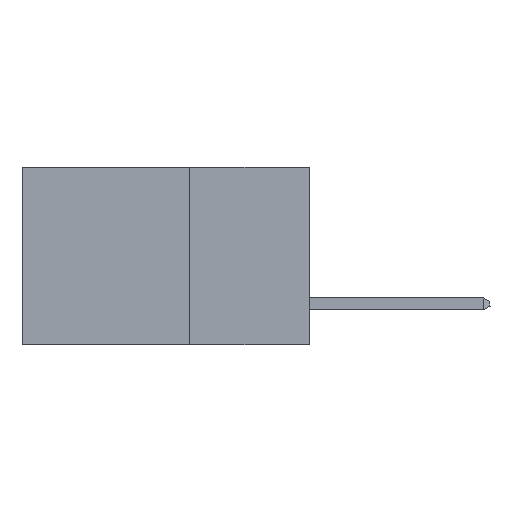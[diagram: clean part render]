
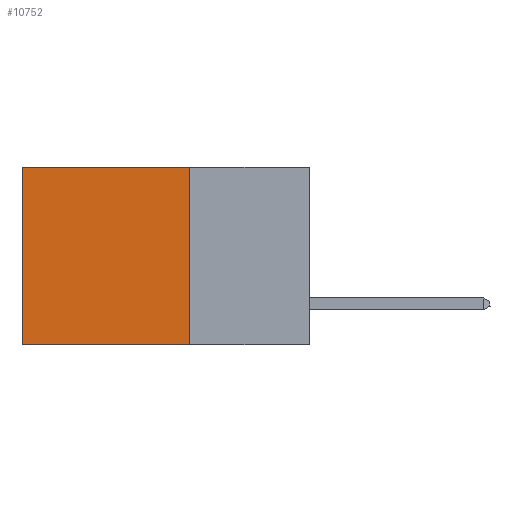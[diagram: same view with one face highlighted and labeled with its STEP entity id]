
A CAD part, left-side view. The second image highlights one B-rep face of the part: STEP entity #10752.
In plain terms, the highlighted planar face has unit normal (-1, 0, 0).
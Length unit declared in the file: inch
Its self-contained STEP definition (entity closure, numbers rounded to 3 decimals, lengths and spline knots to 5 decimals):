
#923 = LINE ( 'NONE', #5842, #4496 ) ;
#1606 = VECTOR ( 'NONE', #9957, 39.37008 ) ;
#1631 = CARTESIAN_POINT ( 'NONE',  ( 0.2875, 0.6, 0. ) ) ;
#1656 = CARTESIAN_POINT ( 'NONE',  ( 0.2875, 0.25, 0. ) ) ;
#2433 = CARTESIAN_POINT ( 'NONE',  ( 0.2875, 0.6, -0.37 ) ) ;
#2585 = LINE ( 'NONE', #5526, #10578 ) ;
#2703 = DIRECTION ( 'NONE',  ( 1., 0., 0. ) ) ;
#2989 = VERTEX_POINT ( 'NONE', #1656 ) ;
#3231 = DIRECTION ( 'NONE',  ( 0., 0., -1. ) ) ;
#3841 = DIRECTION ( 'NONE',  ( 0., 1., 0. ) ) ;
#3977 = CARTESIAN_POINT ( 'NONE',  ( 0.2875, 0.25, -0.37 ) ) ;
#4195 = EDGE_CURVE ( 'NONE', #2989, #6592, #10791, .T. ) ;
#4466 = DIRECTION ( 'NONE',  ( 0., 0., -1. ) ) ;
#4496 = VECTOR ( 'NONE', #3231, 39.37008 ) ;
#5169 = LINE ( 'NONE', #5521, #1606 ) ;
#5521 = CARTESIAN_POINT ( 'NONE',  ( 0.2875, 0.25, 0. ) ) ;
#5526 = CARTESIAN_POINT ( 'NONE',  ( 0.2875, 0.25, -0.37 ) ) ;
#5571 = FACE_OUTER_BOUND ( 'NONE', #9987, .T. ) ;
#5842 = CARTESIAN_POINT ( 'NONE',  ( 0.2875, 0.6, 0. ) ) ;
#5901 = VECTOR ( 'NONE', #6674, 39.37008 ) ;
#5919 = ORIENTED_EDGE ( 'NONE', *, *, #7233, .F. ) ;
#6116 = VERTEX_POINT ( 'NONE', #3977 ) ;
#6592 = VERTEX_POINT ( 'NONE', #1631 ) ;
#6674 = DIRECTION ( 'NONE',  ( 0., 1., 0. ) ) ;
#6745 = ORIENTED_EDGE ( 'NONE', *, *, #7555, .T. ) ;
#6959 = CARTESIAN_POINT ( 'NONE',  ( 0.2875, 0.25, 0. ) ) ;
#7233 = EDGE_CURVE ( 'NONE', #2989, #6116, #5169, .T. ) ;
#7527 = EDGE_CURVE ( 'NONE', #6116, #8042, #2585, .T. ) ;
#7555 = EDGE_CURVE ( 'NONE', #6592, #8042, #923, .T. ) ;
#7877 = AXIS2_PLACEMENT_3D ( 'NONE', #6959, #2703, #4466 ) ;
#7953 = ORIENTED_EDGE ( 'NONE', *, *, #4195, .T. ) ;
#8042 = VERTEX_POINT ( 'NONE', #2433 ) ;
#9172 = ORIENTED_EDGE ( 'NONE', *, *, #7527, .F. ) ;
#9262 = CARTESIAN_POINT ( 'NONE',  ( 0.2875, 0.25, 0. ) ) ;
#9957 = DIRECTION ( 'NONE',  ( 0., 0., -1. ) ) ;
#9987 = EDGE_LOOP ( 'NONE', ( #6745, #9172, #5919, #7953 ) ) ;
#10481 = PLANE ( 'NONE',  #7877 ) ;
#10578 = VECTOR ( 'NONE', #3841, 39.37008 ) ;
#10752 = ADVANCED_FACE ( 'NONE', ( #5571 ), #10481, .F. ) ;
#10791 = LINE ( 'NONE', #9262, #5901 ) ;
